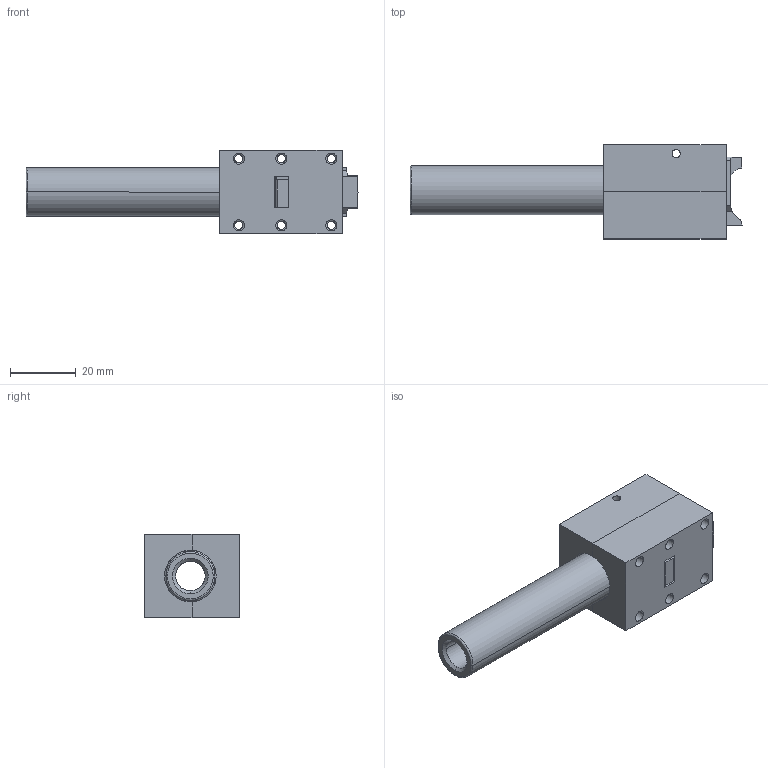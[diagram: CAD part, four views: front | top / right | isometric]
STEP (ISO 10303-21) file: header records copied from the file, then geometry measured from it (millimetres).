
FILE_DESCRIPTION (( 'STEP AP214' ), '1' );
FILE_NAME ('PPDW9 V4 SW9VE Barrel and block.STEP', '2020-12-31T18:39:29', ( '' ), ( '' ), 'SwSTEP 2.0', 'SolidWorks 2020', '' );
FILE_SCHEMA (( 'AUTOMOTIVE_DESIGN' ));
Length unit declared in the file: inch
Products named in the file (4): Barrel Block V4 SM9VE split top; PPDW9 V4 SW9VE Barrel and block; Barrel SW9VE_v1; Barrel Block V4 SM9VE split bottom
Assembly tree (3 placements, depth 2):
  PPDW9 V4 SW9VE Barrel and block
    Barrel SW9VE_v1
    Barrel Block V4 SM9VE split bottom
    Barrel Block V4 SM9VE split top
Bounding box: 101.28 x 28.7 x 25.4 mm (x, y, z)
Volume: 29607.1 mm3; surface area: 18913.2 mm2
Topology: 4 solids, 4 shells, 312 faces, 886 edges, 588 vertices
Faces by surface type: plane 166, bspline 66, cylinder 58, cone 22
Entity records: 15199 total; most frequent: CARTESIAN_POINT 5290, ORIENTED_EDGE 1768, DIRECTION 1265, EDGE_CURVE 884, VERTEX_POINT 588, LINE 529, VECTOR 529, AXIS2_PLACEMENT_3D 368
